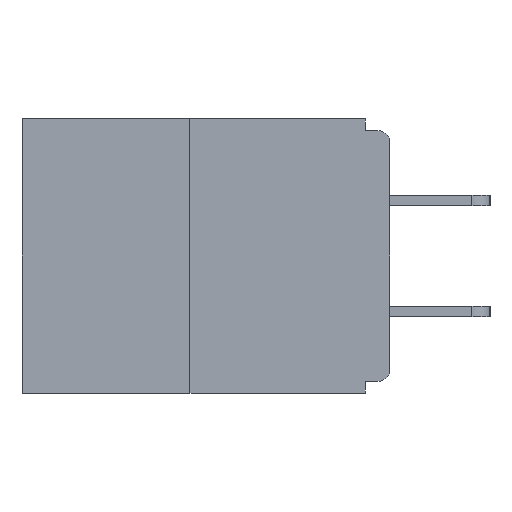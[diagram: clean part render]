
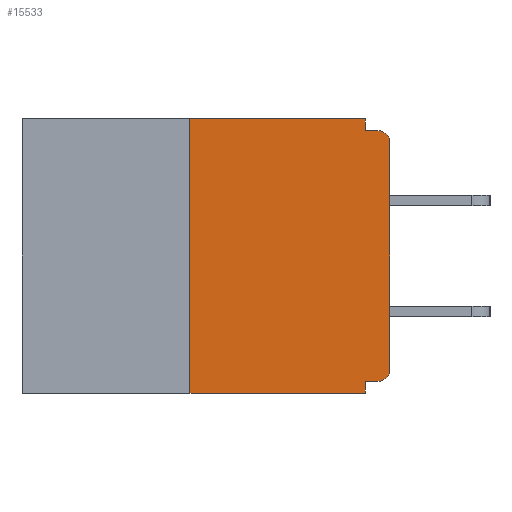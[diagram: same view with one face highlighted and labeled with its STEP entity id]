
A CAD part, left-side view. The second image highlights one B-rep face of the part: STEP entity #15533.
In plain terms, the highlighted planar face has unit normal (-1, 0, 0).
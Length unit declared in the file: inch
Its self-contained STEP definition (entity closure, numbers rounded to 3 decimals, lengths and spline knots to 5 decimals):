
#87 = EDGE_CURVE ( 'NONE', #8511, #10720, #624, .T. ) ;
#559 = VERTEX_POINT ( 'NONE', #12398 ) ;
#624 = CIRCLE ( 'NONE', #12265, 0.015 ) ;
#1272 = ORIENTED_EDGE ( 'NONE', *, *, #15730, .F. ) ;
#1562 = EDGE_CURVE ( 'NONE', #559, #10720, #12012, .T. ) ;
#1629 = ORIENTED_EDGE ( 'NONE', *, *, #87, .T. ) ;
#1933 = LINE ( 'NONE', #9302, #15316 ) ;
#2210 = LINE ( 'NONE', #9349, #2419 ) ;
#2419 = VECTOR ( 'NONE', #15812, 39.37008 ) ;
#2441 = DIRECTION ( 'NONE',  ( 0., -1., 0. ) ) ;
#2669 = VERTEX_POINT ( 'NONE', #10162 ) ;
#3579 = CARTESIAN_POINT ( 'NONE',  ( 0., 0., -0.015 ) ) ;
#3818 = DIRECTION ( 'NONE',  ( 0., 0., -1. ) ) ;
#3890 = CARTESIAN_POINT ( 'NONE',  ( 0., 0.031, -0.343 ) ) ;
#4526 = ORIENTED_EDGE ( 'NONE', *, *, #9042, .T. ) ;
#5036 = CARTESIAN_POINT ( 'NONE',  ( 0., 0., -0.03 ) ) ;
#5337 = FACE_OUTER_BOUND ( 'NONE', #15304, .T. ) ;
#5484 = ORIENTED_EDGE ( 'NONE', *, *, #6212, .F. ) ;
#5799 = LINE ( 'NONE', #10736, #12458 ) ;
#5979 = VECTOR ( 'NONE', #2441, 39.37008 ) ;
#6212 = EDGE_CURVE ( 'NONE', #10958, #12838, #14914, .T. ) ;
#6216 = VERTEX_POINT ( 'NONE', #3890 ) ;
#6314 = CARTESIAN_POINT ( 'NONE',  ( 0., 0., 0. ) ) ;
#6778 = VECTOR ( 'NONE', #7378, 39.37008 ) ;
#6883 = EDGE_CURVE ( 'NONE', #12838, #559, #5799, .T. ) ;
#7016 = AXIS2_PLACEMENT_3D ( 'NONE', #7360, #9865, #8654 ) ;
#7173 = LINE ( 'NONE', #14938, #9230 ) ;
#7274 = VERTEX_POINT ( 'NONE', #14190 ) ;
#7360 = CARTESIAN_POINT ( 'NONE',  ( 0., 0.015, -0.313 ) ) ;
#7378 = DIRECTION ( 'NONE',  ( 0., 0., 1. ) ) ;
#7450 = VERTEX_POINT ( 'NONE', #10722 ) ;
#7686 = DIRECTION ( 'NONE',  ( 1., 0., 0. ) ) ;
#7896 = DIRECTION ( 'NONE',  ( 0., 0., -1. ) ) ;
#8260 = DIRECTION ( 'NONE',  ( 0., -1., 0. ) ) ;
#8511 = VERTEX_POINT ( 'NONE', #5036 ) ;
#8513 = ORIENTED_EDGE ( 'NONE', *, *, #10677, .T. ) ;
#8600 = LINE ( 'NONE', #6314, #6778 ) ;
#8611 = CARTESIAN_POINT ( 'NONE',  ( 0., 0.015, -0.03 ) ) ;
#8654 = DIRECTION ( 'NONE',  ( 0., 0., -1. ) ) ;
#9042 = EDGE_CURVE ( 'NONE', #7274, #7450, #9350, .T. ) ;
#9126 = DIRECTION ( 'NONE',  ( 0., 1., 0. ) ) ;
#9139 = PLANE ( 'NONE',  #13349 ) ;
#9150 = VECTOR ( 'NONE', #9568, 39.37008 ) ;
#9230 = VECTOR ( 'NONE', #13633, 39.37008 ) ;
#9302 = CARTESIAN_POINT ( 'NONE',  ( 0., 0.46, -0.343 ) ) ;
#9349 = CARTESIAN_POINT ( 'NONE',  ( 0., 0.031, -0.343 ) ) ;
#9350 = CIRCLE ( 'NONE', #7016, 0.015 ) ;
#9568 = DIRECTION ( 'NONE',  ( 0., -1., 0. ) ) ;
#9865 = DIRECTION ( 'NONE',  ( -1., 0., 0. ) ) ;
#10162 = CARTESIAN_POINT ( 'NONE',  ( 0., 0.031, -0.328 ) ) ;
#10511 = ORIENTED_EDGE ( 'NONE', *, *, #11096, .F. ) ;
#10529 = VERTEX_POINT ( 'NONE', #12788 ) ;
#10677 = EDGE_CURVE ( 'NONE', #10529, #6216, #1933, .T. ) ;
#10720 = VERTEX_POINT ( 'NONE', #15534 ) ;
#10722 = CARTESIAN_POINT ( 'NONE',  ( 0., 0., -0.313 ) ) ;
#10736 = CARTESIAN_POINT ( 'NONE',  ( 0., 0.031, 0. ) ) ;
#10958 = VERTEX_POINT ( 'NONE', #15495 ) ;
#11096 = EDGE_CURVE ( 'NONE', #2669, #6216, #2210, .T. ) ;
#11409 = CARTESIAN_POINT ( 'NONE',  ( 0., 0., -0.328 ) ) ;
#11501 = DIRECTION ( 'NONE',  ( 0., 0., -1. ) ) ;
#11626 = EDGE_CURVE ( 'NONE', #7450, #8511, #8600, .T. ) ;
#12012 = LINE ( 'NONE', #3579, #9150 ) ;
#12160 = EDGE_CURVE ( 'NONE', #7274, #2669, #13736, .T. ) ;
#12265 = AXIS2_PLACEMENT_3D ( 'NONE', #8611, #14839, #3818 ) ;
#12398 = CARTESIAN_POINT ( 'NONE',  ( 0., 0.031, -0.015 ) ) ;
#12458 = VECTOR ( 'NONE', #7896, 39.37008 ) ;
#12788 = CARTESIAN_POINT ( 'NONE',  ( 0., 0.25, -0.343 ) ) ;
#12838 = VERTEX_POINT ( 'NONE', #14874 ) ;
#12997 = ORIENTED_EDGE ( 'NONE', *, *, #12160, .F. ) ;
#13349 = AXIS2_PLACEMENT_3D ( 'NONE', #14072, #7686, #11501 ) ;
#13633 = DIRECTION ( 'NONE',  ( 0., 0., 1. ) ) ;
#13704 = ORIENTED_EDGE ( 'NONE', *, *, #11626, .T. ) ;
#13736 = LINE ( 'NONE', #11409, #13770 ) ;
#13770 = VECTOR ( 'NONE', #9126, 39.37008 ) ;
#14072 = CARTESIAN_POINT ( 'NONE',  ( 0., 0.46, 0. ) ) ;
#14190 = CARTESIAN_POINT ( 'NONE',  ( 0., 0.015, -0.328 ) ) ;
#14330 = ORIENTED_EDGE ( 'NONE', *, *, #1562, .F. ) ;
#14837 = CARTESIAN_POINT ( 'NONE',  ( 0., 0.46, 0. ) ) ;
#14839 = DIRECTION ( 'NONE',  ( -1., 0., 0. ) ) ;
#14874 = CARTESIAN_POINT ( 'NONE',  ( 0., 0.031, 0. ) ) ;
#14914 = LINE ( 'NONE', #14837, #5979 ) ;
#14938 = CARTESIAN_POINT ( 'NONE',  ( 0., 0.25, 0. ) ) ;
#15304 = EDGE_LOOP ( 'NONE', ( #5484, #1272, #8513, #10511, #12997, #4526, #13704, #1629, #14330, #15399 ) ) ;
#15316 = VECTOR ( 'NONE', #8260, 39.37008 ) ;
#15399 = ORIENTED_EDGE ( 'NONE', *, *, #6883, .F. ) ;
#15495 = CARTESIAN_POINT ( 'NONE',  ( 0., 0.25, 0. ) ) ;
#15533 = ADVANCED_FACE ( 'NONE', ( #5337 ), #9139, .F. ) ;
#15534 = CARTESIAN_POINT ( 'NONE',  ( 0., 0.015, -0.015 ) ) ;
#15730 = EDGE_CURVE ( 'NONE', #10529, #10958, #7173, .T. ) ;
#15812 = DIRECTION ( 'NONE',  ( 0., 0., -1. ) ) ;
